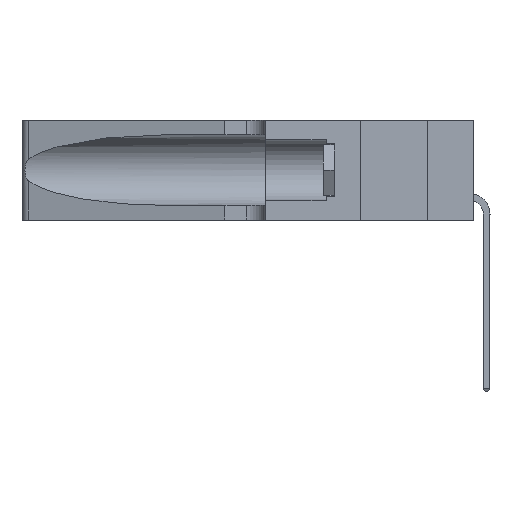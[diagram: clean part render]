
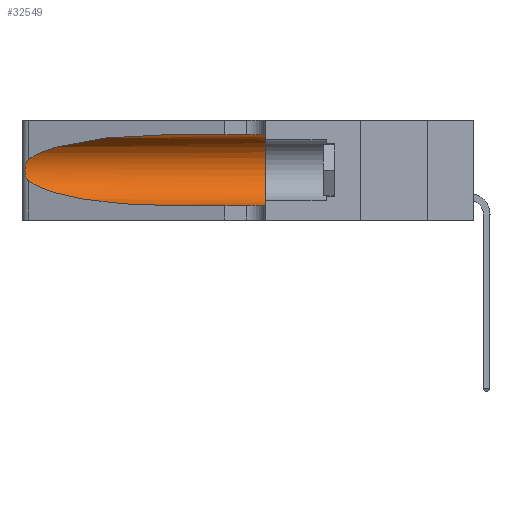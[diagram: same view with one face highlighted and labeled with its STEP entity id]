
A CAD part, left-side view. The second image highlights one B-rep face of the part: STEP entity #32549.
In plain terms, the highlighted cylindrical face has radius 3.308 mm (diameter 6.617 mm), a partial arc.
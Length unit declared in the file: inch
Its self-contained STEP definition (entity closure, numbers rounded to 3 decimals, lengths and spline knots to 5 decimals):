
#69 = VERTEX_POINT ( 'NONE', #3196 ) ;
#2098 = CARTESIAN_POINT ( 'NONE',  ( 0.1305, 1.61858, 0.31525 ) ) ;
#2223 = VERTEX_POINT ( 'NONE', #8906 ) ;
#2914 = CARTESIAN_POINT ( 'NONE',  ( 0.1305, 0.72297, 0.05475 ) ) ;
#3196 = CARTESIAN_POINT ( 'NONE',  ( 0.1305, 0.72297, 0.31525 ) ) ;
#3555 = VECTOR ( 'NONE', #23084, 39.37008 ) ;
#4086 = ORIENTED_EDGE ( 'NONE', *, *, #9585, .T. ) ;
#4509 = ORIENTED_EDGE ( 'NONE', *, *, #15253, .F. ) ;
#5304 = CARTESIAN_POINT ( 'NONE',  ( 0.25487, 1.22718, 0.14631 ) ) ;
#5735 = ORIENTED_EDGE ( 'NONE', *, *, #22784, .T. ) ;
#7209 = EDGE_CURVE ( 'NONE', #69, #17258, #14318, .T. ) ;
#7615 = CARTESIAN_POINT ( 'NONE',  ( 0.25487, 1.22718, 0.22369 ) ) ;
#8511 = LINE ( 'NONE', #22593, #16368 ) ;
#8906 = CARTESIAN_POINT ( 'NONE',  ( 0.1305, 0.35, 0.05475 ) ) ;
#9076 = CARTESIAN_POINT ( 'NONE',  ( 0.26075, 1.23896, 0.19203 ) ) ;
#9193 = CARTESIAN_POINT ( 'NONE',  ( 0.25487, 1.22718, 0.22369 ) ) ;
#9380 = FACE_OUTER_BOUND ( 'NONE', #14916, .T. ) ;
#9585 = EDGE_CURVE ( 'NONE', #69, #25916, #10121, .T. ) ;
#9647 = DIRECTION ( 'NONE',  ( 0., 0., 1. ) ) ;
#10121 =( BOUNDED_CURVE ( )  B_SPLINE_CURVE ( 3, ( #25220, #14642, #16954, #9193 ),
 .UNSPECIFIED., .F., .F. ) 
 B_SPLINE_CURVE_WITH_KNOTS ( ( 4, 4 ),
 ( 1.5708, 2.84003 ),
 .UNSPECIFIED. ) 
 CURVE ( )  GEOMETRIC_REPRESENTATION_ITEM ( )  RATIONAL_B_SPLINE_CURVE ( ( 1., 0.87, 0.87, 1. ) ) 
 REPRESENTATION_ITEM ( '' )  );
#10213 = EDGE_CURVE ( 'NONE', #25916, #22291, #28507, .T. ) ;
#10261 = VERTEX_POINT ( 'NONE', #2914 ) ;
#10505 = ORIENTED_EDGE ( 'NONE', *, *, #10213, .T. ) ;
#11279 = CARTESIAN_POINT ( 'NONE',  ( 0.26018, 1.23835, 0.19895 ) ) ;
#11754 = CARTESIAN_POINT ( 'NONE',  ( 0.26075, 1.23896, 0.178 ) ) ;
#12813 = CARTESIAN_POINT ( 'NONE',  ( 0.1305, 1.61858, 0.185 ) ) ;
#13617 = AXIS2_PLACEMENT_3D ( 'NONE', #12813, #15581, #18137 ) ;
#13915 = CARTESIAN_POINT ( 'NONE',  ( 0.25639, 1.23186, 0.15144 ) ) ;
#14318 = LINE ( 'NONE', #2098, #3555 ) ;
#14642 = CARTESIAN_POINT ( 'NONE',  ( 0.18966, 0.96281, 0.31525 ) ) ;
#14742 = DIRECTION ( 'NONE',  ( 0., -1., 0. ) ) ;
#14916 = EDGE_LOOP ( 'NONE', ( #4086, #10505, #17567, #5735, #4509, #21740 ) ) ;
#15091 = AXIS2_PLACEMENT_3D ( 'NONE', #31367, #16455, #9647 ) ;
#15253 = EDGE_CURVE ( 'NONE', #17258, #2223, #18424, .T. ) ;
#15581 = DIRECTION ( 'NONE',  ( 0., -1., 0. ) ) ;
#16368 = VECTOR ( 'NONE', #14742, 39.37008 ) ;
#16455 = DIRECTION ( 'NONE',  ( 0., 1., 0. ) ) ;
#16827 = CYLINDRICAL_SURFACE ( 'NONE', #13617, 0.13025 ) ;
#16954 = CARTESIAN_POINT ( 'NONE',  ( 0.2373, 1.15595, 0.28018 ) ) ;
#17258 = VERTEX_POINT ( 'NONE', #20164 ) ;
#17567 = ORIENTED_EDGE ( 'NONE', *, *, #30971, .T. ) ;
#18137 = DIRECTION ( 'NONE',  ( 0., 0., -1. ) ) ;
#18424 = CIRCLE ( 'NONE', #15091, 0.13025 ) ;
#19250 = CARTESIAN_POINT ( 'NONE',  ( 0.25555, 1.22993, 0.14849 ) ) ;
#20164 = CARTESIAN_POINT ( 'NONE',  ( 0.1305, 0.35, 0.31525 ) ) ;
#21740 = ORIENTED_EDGE ( 'NONE', *, *, #7209, .F. ) ;
#21884 = CARTESIAN_POINT ( 'NONE',  ( 0.25856, 1.23593, 0.16098 ) ) ;
#21908 = CARTESIAN_POINT ( 'NONE',  ( 0.25487, 1.22718, 0.14631 ) ) ;
#22291 = VERTEX_POINT ( 'NONE', #5304 ) ;
#22593 = CARTESIAN_POINT ( 'NONE',  ( 0.1305, 1.61858, 0.05475 ) ) ;
#22784 = EDGE_CURVE ( 'NONE', #10261, #2223, #8511, .T. ) ;
#23084 = DIRECTION ( 'NONE',  ( 0., -1., 0. ) ) ;
#23844 = CARTESIAN_POINT ( 'NONE',  ( 0.25789, 1.23486, 0.15765 ) ) ;
#23852 = CARTESIAN_POINT ( 'NONE',  ( 0.1305, 0.72297, 0.05475 ) ) ;
#24873 = CARTESIAN_POINT ( 'NONE',  ( 0.25639, 1.23184, 0.21858 ) ) ;
#25220 = CARTESIAN_POINT ( 'NONE',  ( 0.1305, 0.72297, 0.31525 ) ) ;
#25916 = VERTEX_POINT ( 'NONE', #7615 ) ;
#27048 = CARTESIAN_POINT ( 'NONE',  ( 0.25487, 1.22718, 0.22369 ) ) ;
#27515 = CARTESIAN_POINT ( 'NONE',  ( 0.25555, 1.22994, 0.2215 ) ) ;
#28235 = CARTESIAN_POINT ( 'NONE',  ( 0.2373, 1.15595, 0.08982 ) ) ;
#28507 = B_SPLINE_CURVE_WITH_KNOTS ( 'NONE', 3,
 ( #27048, #27515, #24873, #30014, #29650, #11279, #9076, #11754, #32282, #21884, #23844, #13915, #19250, #21908 ),
 .UNSPECIFIED., .F., .F.,
 ( 4, 2, 2, 2, 2, 2, 4 ),
 ( 0., 0.00027, 0.00053, 0.00107, 0.0016, 0.00187, 0.00214 ),
 .UNSPECIFIED. ) ;
#29222 = CARTESIAN_POINT ( 'NONE',  ( 0.18966, 0.96281, 0.05475 ) ) ;
#29650 = CARTESIAN_POINT ( 'NONE',  ( 0.25854, 1.2359, 0.20912 ) ) ;
#29942 =( BOUNDED_CURVE ( )  B_SPLINE_CURVE ( 3, ( #33208, #28235, #29222, #23852 ),
 .UNSPECIFIED., .F., .F. ) 
 B_SPLINE_CURVE_WITH_KNOTS ( ( 4, 4 ),
 ( 3.44316, 4.71239 ),
 .UNSPECIFIED. ) 
 CURVE ( )  GEOMETRIC_REPRESENTATION_ITEM ( )  RATIONAL_B_SPLINE_CURVE ( ( 1., 0.87, 0.87, 1. ) ) 
 REPRESENTATION_ITEM ( '' )  );
#30014 = CARTESIAN_POINT ( 'NONE',  ( 0.25787, 1.23484, 0.2124 ) ) ;
#30971 = EDGE_CURVE ( 'NONE', #22291, #10261, #29942, .T. ) ;
#31367 = CARTESIAN_POINT ( 'NONE',  ( 0.1305, 0.35, 0.185 ) ) ;
#32282 = CARTESIAN_POINT ( 'NONE',  ( 0.26017, 1.23833, 0.17102 ) ) ;
#32549 = ADVANCED_FACE ( 'NONE', ( #9380 ), #16827, .F. ) ;
#33208 = CARTESIAN_POINT ( 'NONE',  ( 0.25487, 1.22718, 0.14631 ) ) ;
